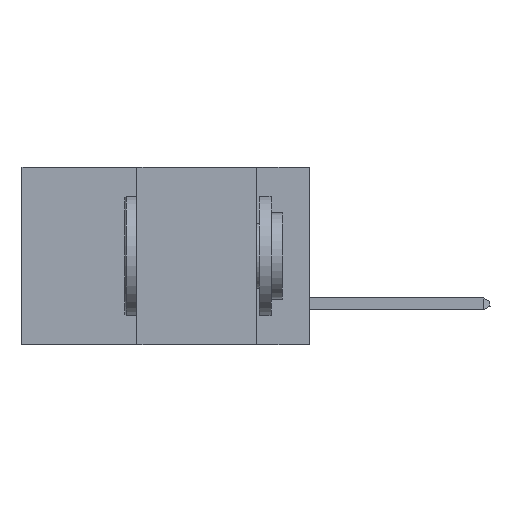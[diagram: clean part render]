
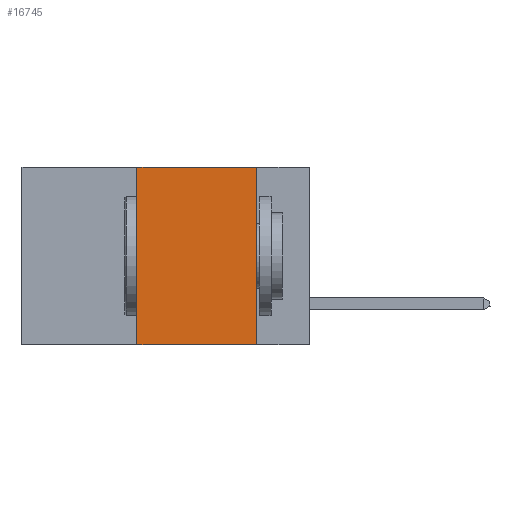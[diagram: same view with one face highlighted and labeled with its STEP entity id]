
A CAD part, left-side view. The second image highlights one B-rep face of the part: STEP entity #16745.
In plain terms, the highlighted planar face has unit normal (-1, 0, 0).
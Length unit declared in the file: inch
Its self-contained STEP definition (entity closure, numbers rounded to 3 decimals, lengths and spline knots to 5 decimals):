
#852 = AXIS2_PLACEMENT_3D ( 'NONE', #26908, #5511, #7499 ) ;
#2279 = VECTOR ( 'NONE', #5334, 39.37008 ) ;
#2562 = EDGE_CURVE ( 'NONE', #8791, #21213, #27009, .T. ) ;
#4168 = DIRECTION ( 'NONE',  ( 0., 0., 1. ) ) ;
#4904 = DIRECTION ( 'NONE',  ( 0., 0., -1. ) ) ;
#5334 = DIRECTION ( 'NONE',  ( 0., -1., 0. ) ) ;
#5511 = DIRECTION ( 'NONE',  ( 1., 0., 0. ) ) ;
#7499 = DIRECTION ( 'NONE',  ( 0., 0., -1. ) ) ;
#8257 = EDGE_CURVE ( 'NONE', #21213, #20815, #19832, .T. ) ;
#8290 = ORIENTED_EDGE ( 'NONE', *, *, #12857, .T. ) ;
#8602 = CARTESIAN_POINT ( 'NONE',  ( 0., 0.36, -0.37 ) ) ;
#8791 = VERTEX_POINT ( 'NONE', #8602 ) ;
#9025 = CARTESIAN_POINT ( 'NONE',  ( 0., 0.6, -0.37 ) ) ;
#9636 = CARTESIAN_POINT ( 'NONE',  ( 0., 0.6, 0. ) ) ;
#10817 = CARTESIAN_POINT ( 'NONE',  ( 0., 0.36, 0. ) ) ;
#11708 = PLANE ( 'NONE',  #852 ) ;
#12830 = CARTESIAN_POINT ( 'NONE',  ( 0., 0.36, 0. ) ) ;
#12857 = EDGE_CURVE ( 'NONE', #8791, #13074, #20810, .T. ) ;
#13074 = VERTEX_POINT ( 'NONE', #19243 ) ;
#13751 = EDGE_LOOP ( 'NONE', ( #19483, #21421, #22757, #8290 ) ) ;
#14624 = EDGE_CURVE ( 'NONE', #20815, #13074, #18725, .T. ) ;
#16745 = ADVANCED_FACE ( 'NONE', ( #27231 ), #11708, .F. ) ;
#17832 = CARTESIAN_POINT ( 'NONE',  ( 0., 0.11, 0. ) ) ;
#18381 = VECTOR ( 'NONE', #4904, 39.37008 ) ;
#18725 = LINE ( 'NONE', #17832, #18381 ) ;
#19243 = CARTESIAN_POINT ( 'NONE',  ( 0., 0.11, -0.37 ) ) ;
#19483 = ORIENTED_EDGE ( 'NONE', *, *, #14624, .F. ) ;
#19832 = LINE ( 'NONE', #9636, #2279 ) ;
#20514 = VECTOR ( 'NONE', #4168, 39.37008 ) ;
#20810 = LINE ( 'NONE', #9025, #24558 ) ;
#20815 = VERTEX_POINT ( 'NONE', #22955 ) ;
#21213 = VERTEX_POINT ( 'NONE', #10817 ) ;
#21421 = ORIENTED_EDGE ( 'NONE', *, *, #8257, .F. ) ;
#22747 = DIRECTION ( 'NONE',  ( 0., -1., 0. ) ) ;
#22757 = ORIENTED_EDGE ( 'NONE', *, *, #2562, .F. ) ;
#22955 = CARTESIAN_POINT ( 'NONE',  ( 0., 0.11, 0. ) ) ;
#24558 = VECTOR ( 'NONE', #22747, 39.37008 ) ;
#26908 = CARTESIAN_POINT ( 'NONE',  ( 0., 0.6, 0. ) ) ;
#27009 = LINE ( 'NONE', #12830, #20514 ) ;
#27231 = FACE_OUTER_BOUND ( 'NONE', #13751, .T. ) ;
